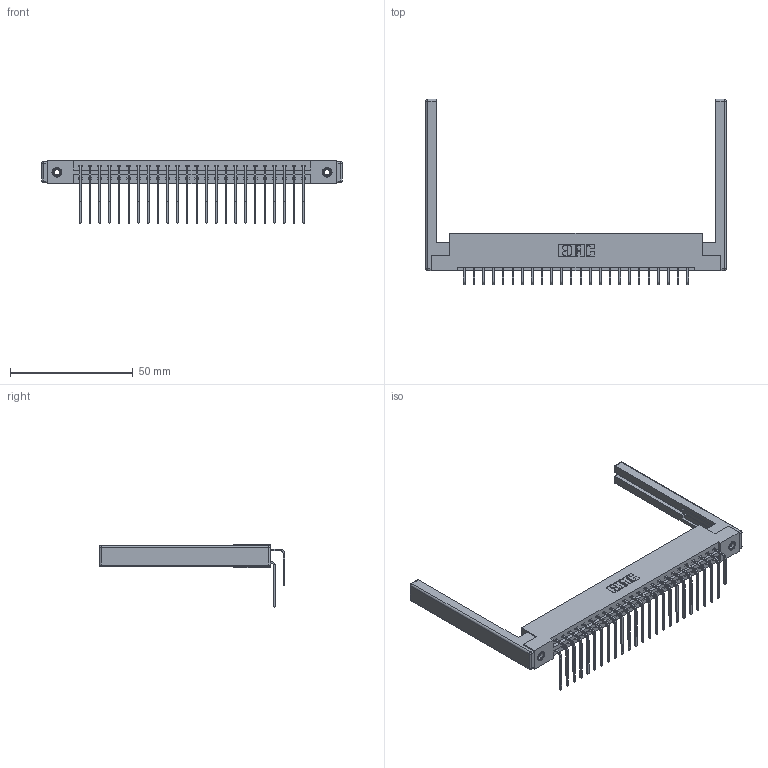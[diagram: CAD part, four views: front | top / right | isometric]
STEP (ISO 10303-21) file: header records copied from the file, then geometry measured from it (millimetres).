
FILE_DESCRIPTION (( 'STEP AP203' ), '1' );
FILE_NAME ('337-048-559-268.STEP', '2019-10-09T15:18:41', ( '' ), ( '' ), 'SwSTEP 2.0', 'SolidWorks 2016', '' );
FILE_SCHEMA (( 'CONFIG_CONTROL_DESIGN' ));
Length unit declared in the file: inch
Products named in the file (6): 345-250-001_345-250-001-102; 345-292-001_559 Tail - 2; 337 Part_Flush Mounting Lugs - 0.156 Dia-TI; 345-292-001_558 559 Tail - 1; 337-048-559-268; 307-220-068
Assembly tree (53 placements, depth 2):
  337-048-559-268
    337 Part_Flush Mounting Lugs - 0.156 Dia-TI
    345-292-001_558 559 Tail - 1  x24
    345-292-001_559 Tail - 2  x24
    345-250-001_345-250-001-102  x2
    307-220-068  x2
Bounding box: 122.53 x 75.63 x 25.53 mm (x, y, z)
Volume: 17335.2 mm3; surface area: 19890.4 mm2
Topology: 53 solids, 53 shells, 2956 faces, 8717 edges, 5726 vertices
Faces by surface type: plane 2078, cylinder 854, cone 12, sphere 8, torus 4
Entity records: 25480 total; most frequent: CARTESIAN_POINT 4318, ORIENTED_EDGE 4192, DIRECTION 3758, EDGE_CURVE 2096, VECTOR 1878, LINE 1878, VERTEX_POINT 1386, AXIS2_PLACEMENT_3D 940
